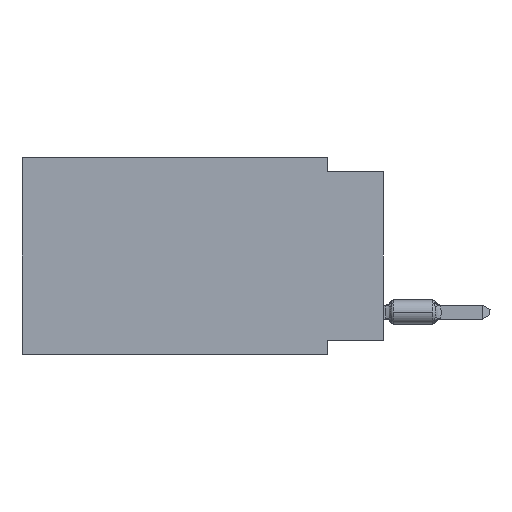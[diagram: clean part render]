
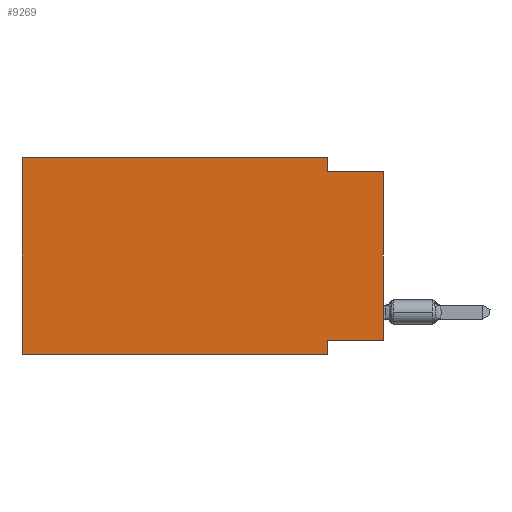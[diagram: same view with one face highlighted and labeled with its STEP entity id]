
A CAD part, left-side view. The second image highlights one B-rep face of the part: STEP entity #9269.
In plain terms, the highlighted planar face has unit normal (-1, 0, 0).
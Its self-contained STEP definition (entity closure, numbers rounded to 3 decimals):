
#24 = LINE ( 'NONE', #8135, #19147 ) ;
#549 = LINE ( 'NONE', #9815, #25378 ) ;
#816 = ORIENTED_EDGE ( 'NONE', *, *, #19872, .T. ) ;
#1354 = DIRECTION ( 'NONE',  ( 0., -1., 0. ) ) ;
#2411 = VECTOR ( 'NONE', #37739, 1000. ) ;
#2443 = VERTEX_POINT ( 'NONE', #23814 ) ;
#3023 = AXIS2_PLACEMENT_3D ( 'NONE', #24776, #6806, #6996 ) ;
#3141 = CARTESIAN_POINT ( 'NONE',  ( 0., 2.54, -8.89 ) ) ;
#3267 = EDGE_CURVE ( 'NONE', #31968, #28543, #10043, .T. ) ;
#3534 = FACE_OUTER_BOUND ( 'NONE', #30912, .T. ) ;
#3762 = CARTESIAN_POINT ( 'NONE',  ( 0., 0., -8.255 ) ) ;
#4253 = EDGE_CURVE ( 'NONE', #19873, #31968, #24, .T. ) ;
#5182 = ORIENTED_EDGE ( 'NONE', *, *, #10156, .F. ) ;
#5952 = CARTESIAN_POINT ( 'NONE',  ( 0., 2.54, -8.89 ) ) ;
#6806 = DIRECTION ( 'NONE',  ( 1., 0., 0. ) ) ;
#6996 = DIRECTION ( 'NONE',  ( 0., 0., -1. ) ) ;
#7083 = VECTOR ( 'NONE', #22015, 1000. ) ;
#8135 = CARTESIAN_POINT ( 'NONE',  ( 0., 16.383, 0. ) ) ;
#8182 = LINE ( 'NONE', #34662, #13932 ) ;
#8705 = CARTESIAN_POINT ( 'NONE',  ( 0., 0., -0.635 ) ) ;
#9203 = VERTEX_POINT ( 'NONE', #3141 ) ;
#9220 = EDGE_CURVE ( 'NONE', #35822, #22347, #35617, .T. ) ;
#9247 = VECTOR ( 'NONE', #15322, 1000. ) ;
#9269 = ADVANCED_FACE ( 'NONE', ( #3534 ), #20935, .F. ) ;
#9815 = CARTESIAN_POINT ( 'NONE',  ( 0., 0., -8.255 ) ) ;
#10043 = LINE ( 'NONE', #30738, #30488 ) ;
#10156 = EDGE_CURVE ( 'NONE', #2443, #9203, #20842, .T. ) ;
#12183 = ORIENTED_EDGE ( 'NONE', *, *, #4253, .F. ) ;
#13932 = VECTOR ( 'NONE', #34110, 1000. ) ;
#15322 = DIRECTION ( 'NONE',  ( 0., 0., 1. ) ) ;
#15892 = CARTESIAN_POINT ( 'NONE',  ( 0., 0., 0. ) ) ;
#18082 = ORIENTED_EDGE ( 'NONE', *, *, #26738, .T. ) ;
#19147 = VECTOR ( 'NONE', #19949, 1000. ) ;
#19792 = CARTESIAN_POINT ( 'NONE',  ( 0., 16.383, 0. ) ) ;
#19872 = EDGE_CURVE ( 'NONE', #33139, #22347, #30204, .T. ) ;
#19873 = VERTEX_POINT ( 'NONE', #33282 ) ;
#19949 = DIRECTION ( 'NONE',  ( 0., 0., 1. ) ) ;
#20842 = LINE ( 'NONE', #5952, #21610 ) ;
#20935 = PLANE ( 'NONE',  #3023 ) ;
#21610 = VECTOR ( 'NONE', #32816, 1000. ) ;
#21626 = DIRECTION ( 'NONE',  ( 0., 1., 0. ) ) ;
#22015 = DIRECTION ( 'NONE',  ( 0., 0., -1. ) ) ;
#22347 = VERTEX_POINT ( 'NONE', #8705 ) ;
#23418 = CARTESIAN_POINT ( 'NONE',  ( 0., 2.54, 0. ) ) ;
#23814 = CARTESIAN_POINT ( 'NONE',  ( 0., 2.54, -8.255 ) ) ;
#24776 = CARTESIAN_POINT ( 'NONE',  ( 0., 16.383, 0. ) ) ;
#25340 = EDGE_CURVE ( 'NONE', #28543, #35822, #27626, .T. ) ;
#25378 = VECTOR ( 'NONE', #21626, 1000. ) ;
#26535 = CARTESIAN_POINT ( 'NONE',  ( 0., 0., -0.635 ) ) ;
#26738 = EDGE_CURVE ( 'NONE', #19873, #9203, #8182, .T. ) ;
#27626 = LINE ( 'NONE', #34364, #7083 ) ;
#27710 = ORIENTED_EDGE ( 'NONE', *, *, #3267, .F. ) ;
#27897 = ORIENTED_EDGE ( 'NONE', *, *, #9220, .F. ) ;
#28543 = VERTEX_POINT ( 'NONE', #23418 ) ;
#29530 = ORIENTED_EDGE ( 'NONE', *, *, #25340, .F. ) ;
#30204 = LINE ( 'NONE', #15892, #9247 ) ;
#30488 = VECTOR ( 'NONE', #1354, 1000. ) ;
#30738 = CARTESIAN_POINT ( 'NONE',  ( 0., 16.383, 0. ) ) ;
#30912 = EDGE_LOOP ( 'NONE', ( #816, #27897, #29530, #27710, #12183, #18082, #5182, #34030 ) ) ;
#31968 = VERTEX_POINT ( 'NONE', #19792 ) ;
#32816 = DIRECTION ( 'NONE',  ( 0., 0., -1. ) ) ;
#32978 = EDGE_CURVE ( 'NONE', #33139, #2443, #549, .T. ) ;
#33139 = VERTEX_POINT ( 'NONE', #3762 ) ;
#33282 = CARTESIAN_POINT ( 'NONE',  ( 0., 16.383, -8.89 ) ) ;
#34015 = CARTESIAN_POINT ( 'NONE',  ( 0., 2.54, -0.635 ) ) ;
#34030 = ORIENTED_EDGE ( 'NONE', *, *, #32978, .F. ) ;
#34110 = DIRECTION ( 'NONE',  ( 0., -1., 0. ) ) ;
#34364 = CARTESIAN_POINT ( 'NONE',  ( 0., 2.54, 0. ) ) ;
#34662 = CARTESIAN_POINT ( 'NONE',  ( 0., 16.383, -8.89 ) ) ;
#35617 = LINE ( 'NONE', #26535, #2411 ) ;
#35822 = VERTEX_POINT ( 'NONE', #34015 ) ;
#37739 = DIRECTION ( 'NONE',  ( 0., -1., 0. ) ) ;
